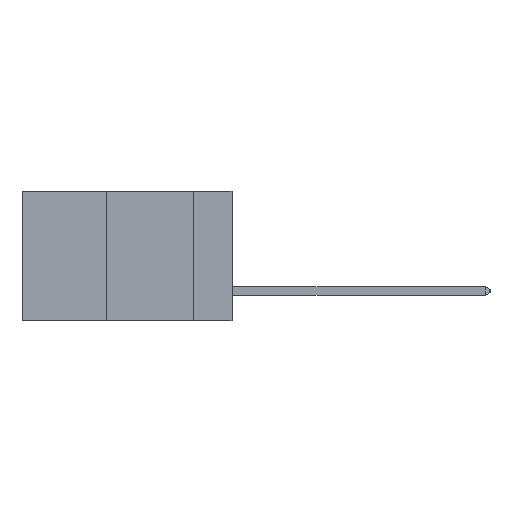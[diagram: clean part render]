
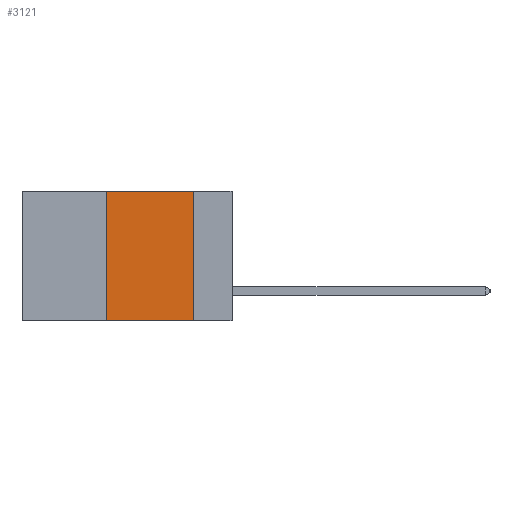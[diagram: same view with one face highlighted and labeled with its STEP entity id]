
A CAD part, left-side view. The second image highlights one B-rep face of the part: STEP entity #3121.
In plain terms, the highlighted planar face has unit normal (-1, 0, 0).
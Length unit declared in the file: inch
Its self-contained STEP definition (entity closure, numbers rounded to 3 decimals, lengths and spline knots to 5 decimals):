
#117 = CARTESIAN_POINT ( 'NONE',  ( 0., 0.11, -0.37 ) ) ;
#462 = VERTEX_POINT ( 'NONE', #7463 ) ;
#1093 = CARTESIAN_POINT ( 'NONE',  ( 0., 0.11, 0. ) ) ;
#1208 = CARTESIAN_POINT ( 'NONE',  ( 0., 0.36, 0. ) ) ;
#2478 = DIRECTION ( 'NONE',  ( 0., 0., 1. ) ) ;
#2665 = ORIENTED_EDGE ( 'NONE', *, *, #13785, .F. ) ;
#3121 = ADVANCED_FACE ( 'NONE', ( #13191 ), #12926, .F. ) ;
#3283 = VERTEX_POINT ( 'NONE', #117 ) ;
#4085 = CARTESIAN_POINT ( 'NONE',  ( 0., 0.11, 0. ) ) ;
#4370 = CARTESIAN_POINT ( 'NONE',  ( 0., 0.6, -0.37 ) ) ;
#5502 = EDGE_LOOP ( 'NONE', ( #13740, #2665, #7683, #14299 ) ) ;
#5833 = CARTESIAN_POINT ( 'NONE',  ( 0., 0.6, 0. ) ) ;
#5958 = VERTEX_POINT ( 'NONE', #1093 ) ;
#7025 = DIRECTION ( 'NONE',  ( 1., 0., 0. ) ) ;
#7463 = CARTESIAN_POINT ( 'NONE',  ( 0., 0.36, 0. ) ) ;
#7512 = EDGE_CURVE ( 'NONE', #9660, #3283, #15652, .T. ) ;
#7683 = ORIENTED_EDGE ( 'NONE', *, *, #9098, .F. ) ;
#7960 = DIRECTION ( 'NONE',  ( 0., -1., 0. ) ) ;
#8958 = VECTOR ( 'NONE', #10262, 39.37008 ) ;
#9069 = VECTOR ( 'NONE', #14796, 39.37008 ) ;
#9098 = EDGE_CURVE ( 'NONE', #9660, #462, #11475, .T. ) ;
#9425 = AXIS2_PLACEMENT_3D ( 'NONE', #5833, #7025, #15325 ) ;
#9660 = VERTEX_POINT ( 'NONE', #13170 ) ;
#9893 = EDGE_CURVE ( 'NONE', #5958, #3283, #15390, .T. ) ;
#10262 = DIRECTION ( 'NONE',  ( 0., -1., 0. ) ) ;
#11377 = CARTESIAN_POINT ( 'NONE',  ( 0., 0.6, 0. ) ) ;
#11475 = LINE ( 'NONE', #1208, #14301 ) ;
#12094 = LINE ( 'NONE', #11377, #8958 ) ;
#12479 = VECTOR ( 'NONE', #7960, 39.37008 ) ;
#12926 = PLANE ( 'NONE',  #9425 ) ;
#13170 = CARTESIAN_POINT ( 'NONE',  ( 0., 0.36, -0.37 ) ) ;
#13191 = FACE_OUTER_BOUND ( 'NONE', #5502, .T. ) ;
#13740 = ORIENTED_EDGE ( 'NONE', *, *, #9893, .F. ) ;
#13785 = EDGE_CURVE ( 'NONE', #462, #5958, #12094, .T. ) ;
#14299 = ORIENTED_EDGE ( 'NONE', *, *, #7512, .T. ) ;
#14301 = VECTOR ( 'NONE', #2478, 39.37008 ) ;
#14796 = DIRECTION ( 'NONE',  ( 0., 0., -1. ) ) ;
#15325 = DIRECTION ( 'NONE',  ( 0., 0., -1. ) ) ;
#15390 = LINE ( 'NONE', #4085, #9069 ) ;
#15652 = LINE ( 'NONE', #4370, #12479 ) ;
